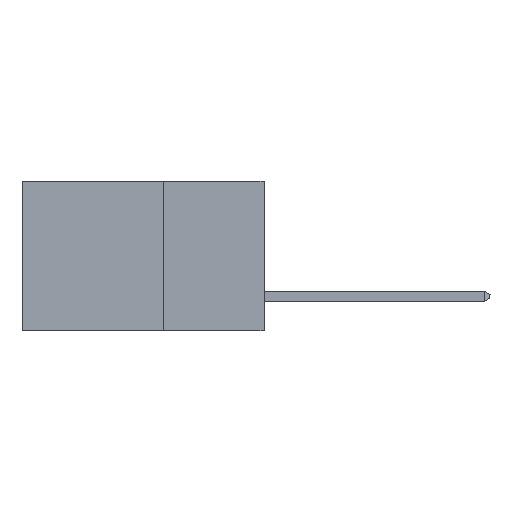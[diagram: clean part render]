
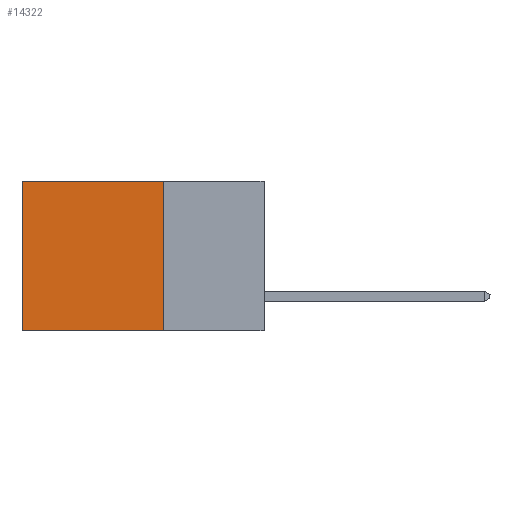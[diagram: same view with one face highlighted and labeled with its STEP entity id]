
A CAD part, left-side view. The second image highlights one B-rep face of the part: STEP entity #14322.
In plain terms, the highlighted planar face has unit normal (-1, 0, 0).
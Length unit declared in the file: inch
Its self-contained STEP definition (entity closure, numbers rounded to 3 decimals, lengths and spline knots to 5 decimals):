
#1687 = DIRECTION ( 'NONE',  ( 0., 0., -1. ) ) ;
#1763 = LINE ( 'NONE', #3202, #14746 ) ;
#1995 = EDGE_CURVE ( 'NONE', #9880, #13097, #13430, .T. ) ;
#3202 = CARTESIAN_POINT ( 'NONE',  ( 0.2615, 0.25, 0. ) ) ;
#3371 = ORIENTED_EDGE ( 'NONE', *, *, #10280, .T. ) ;
#3652 = CARTESIAN_POINT ( 'NONE',  ( 0.2615, 0.25, -0.37 ) ) ;
#4078 = CARTESIAN_POINT ( 'NONE',  ( 0.2615, 0.25, 0. ) ) ;
#4100 = VECTOR ( 'NONE', #8875, 39.37008 ) ;
#4143 = FACE_OUTER_BOUND ( 'NONE', #12683, .T. ) ;
#4163 = VERTEX_POINT ( 'NONE', #4078 ) ;
#4169 = EDGE_CURVE ( 'NONE', #4163, #11755, #1763, .T. ) ;
#4259 = CARTESIAN_POINT ( 'NONE',  ( 0.2615, 0.6, -0.37 ) ) ;
#4732 = AXIS2_PLACEMENT_3D ( 'NONE', #7559, #12377, #1687 ) ;
#5023 = ORIENTED_EDGE ( 'NONE', *, *, #1995, .F. ) ;
#6236 = CARTESIAN_POINT ( 'NONE',  ( 0.2615, 0.6, 0. ) ) ;
#6535 = LINE ( 'NONE', #12331, #4100 ) ;
#6761 = CARTESIAN_POINT ( 'NONE',  ( 0.2615, 0.25, -0.37 ) ) ;
#7559 = CARTESIAN_POINT ( 'NONE',  ( 0.2615, 0.25, -0.37 ) ) ;
#8050 = VECTOR ( 'NONE', #13710, 39.37008 ) ;
#8135 = EDGE_CURVE ( 'NONE', #4163, #9880, #6535, .T. ) ;
#8784 = DIRECTION ( 'NONE',  ( 0., 1., 0. ) ) ;
#8875 = DIRECTION ( 'NONE',  ( 0., 0., -1. ) ) ;
#9880 = VERTEX_POINT ( 'NONE', #3652 ) ;
#10280 = EDGE_CURVE ( 'NONE', #11755, #13097, #14725, .T. ) ;
#10401 = CARTESIAN_POINT ( 'NONE',  ( 0.2615, 0.6, -0.37 ) ) ;
#11172 = ORIENTED_EDGE ( 'NONE', *, *, #8135, .F. ) ;
#11755 = VERTEX_POINT ( 'NONE', #6236 ) ;
#12331 = CARTESIAN_POINT ( 'NONE',  ( 0.2615, 0.25, -0.37 ) ) ;
#12377 = DIRECTION ( 'NONE',  ( 1., 0., 0. ) ) ;
#12495 = DIRECTION ( 'NONE',  ( 0., 0., -1. ) ) ;
#12683 = EDGE_LOOP ( 'NONE', ( #3371, #5023, #11172, #13028 ) ) ;
#13028 = ORIENTED_EDGE ( 'NONE', *, *, #4169, .T. ) ;
#13097 = VERTEX_POINT ( 'NONE', #10401 ) ;
#13430 = LINE ( 'NONE', #6761, #8050 ) ;
#13710 = DIRECTION ( 'NONE',  ( 0., 1., 0. ) ) ;
#14322 = ADVANCED_FACE ( 'NONE', ( #4143 ), #14531, .F. ) ;
#14531 = PLANE ( 'NONE',  #4732 ) ;
#14603 = VECTOR ( 'NONE', #12495, 39.37008 ) ;
#14725 = LINE ( 'NONE', #4259, #14603 ) ;
#14746 = VECTOR ( 'NONE', #8784, 39.37008 ) ;
